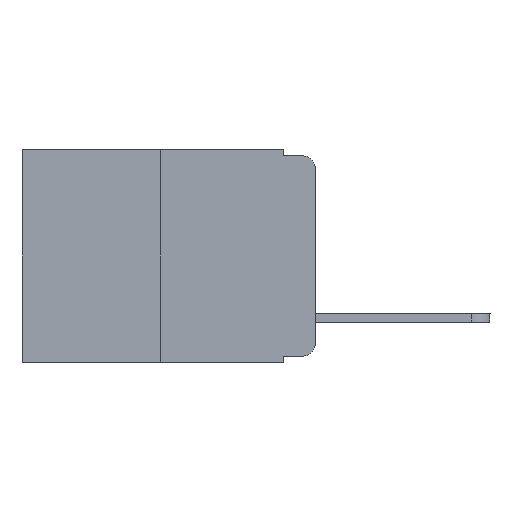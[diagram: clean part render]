
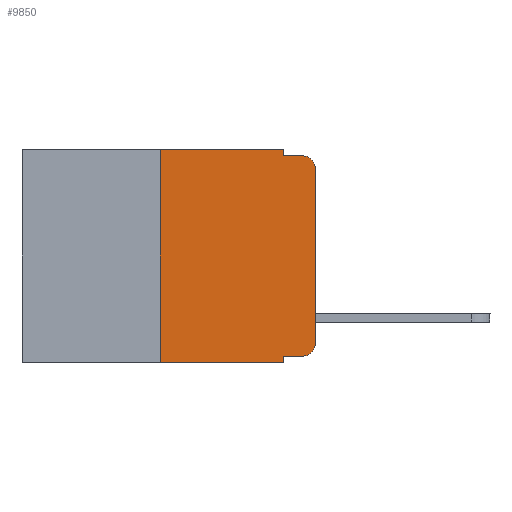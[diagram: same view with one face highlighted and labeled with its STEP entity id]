
A CAD part, left-side view. The second image highlights one B-rep face of the part: STEP entity #9850.
In plain terms, the highlighted planar face has unit normal (-1, 0, 0).
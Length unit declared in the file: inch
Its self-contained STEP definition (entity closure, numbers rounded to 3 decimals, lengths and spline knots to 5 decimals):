
#10 = ORIENTED_EDGE ( 'NONE', *, *, #16839, .T. ) ;
#225 = ORIENTED_EDGE ( 'NONE', *, *, #1136, .F. ) ;
#722 = CARTESIAN_POINT ( 'NONE',  ( 0., 0.02, -0.313 ) ) ;
#817 = DIRECTION ( 'NONE',  ( 0., 0., -1. ) ) ;
#880 = ORIENTED_EDGE ( 'NONE', *, *, #20250, .F. ) ;
#1073 = CARTESIAN_POINT ( 'NONE',  ( 0., 0., -0.313 ) ) ;
#1102 = EDGE_CURVE ( 'NONE', #17290, #2935, #16738, .T. ) ;
#1136 = EDGE_CURVE ( 'NONE', #17198, #19811, #17322, .T. ) ;
#1626 = VECTOR ( 'NONE', #12960, 39.37008 ) ;
#1809 = DIRECTION ( 'NONE',  ( 0., 0., -1. ) ) ;
#1826 = VERTEX_POINT ( 'NONE', #2982 ) ;
#2339 = CARTESIAN_POINT ( 'NONE',  ( 0., 0.051, -0.333 ) ) ;
#2357 = VECTOR ( 'NONE', #1809, 39.37008 ) ;
#2485 = EDGE_CURVE ( 'NONE', #13202, #9995, #9866, .T. ) ;
#2821 = EDGE_CURVE ( 'NONE', #19811, #8246, #12949, .T. ) ;
#2871 = AXIS2_PLACEMENT_3D ( 'NONE', #7156, #5715, #10146 ) ;
#2935 = VERTEX_POINT ( 'NONE', #4811 ) ;
#2982 = CARTESIAN_POINT ( 'NONE',  ( 0., 0.02, -0.333 ) ) ;
#3121 = CARTESIAN_POINT ( 'NONE',  ( 0., 0.051, -0.01 ) ) ;
#3383 = EDGE_CURVE ( 'NONE', #13202, #17198, #8589, .T. ) ;
#3696 = ORIENTED_EDGE ( 'NONE', *, *, #3383, .F. ) ;
#4072 = AXIS2_PLACEMENT_3D ( 'NONE', #7549, #15068, #19740 ) ;
#4455 = CIRCLE ( 'NONE', #16898, 0.02 ) ;
#4811 = CARTESIAN_POINT ( 'NONE',  ( 0., 0., -0.03 ) ) ;
#4824 = CARTESIAN_POINT ( 'NONE',  ( 0., 0.473, -0.343 ) ) ;
#4958 = LINE ( 'NONE', #11219, #12632 ) ;
#5237 = VECTOR ( 'NONE', #817, 39.37008 ) ;
#5255 = ORIENTED_EDGE ( 'NONE', *, *, #5958, .T. ) ;
#5276 = VECTOR ( 'NONE', #18372, 39.37008 ) ;
#5350 = LINE ( 'NONE', #2339, #8603 ) ;
#5715 = DIRECTION ( 'NONE',  ( -1., 0., 0. ) ) ;
#5958 = EDGE_CURVE ( 'NONE', #2935, #11087, #12752, .T. ) ;
#7139 = CARTESIAN_POINT ( 'NONE',  ( 0., 0.25, -0.343 ) ) ;
#7156 = CARTESIAN_POINT ( 'NONE',  ( 0., 0.02, -0.03 ) ) ;
#7549 = CARTESIAN_POINT ( 'NONE',  ( 0., 0.473, 0. ) ) ;
#8246 = VERTEX_POINT ( 'NONE', #3121 ) ;
#8589 = LINE ( 'NONE', #13322, #9729 ) ;
#8603 = VECTOR ( 'NONE', #14796, 39.37008 ) ;
#8794 = FACE_OUTER_BOUND ( 'NONE', #15104, .T. ) ;
#8991 = PLANE ( 'NONE',  #4072 ) ;
#9330 = CARTESIAN_POINT ( 'NONE',  ( 0., 0.473, 0. ) ) ;
#9729 = VECTOR ( 'NONE', #16395, 39.37008 ) ;
#9737 = CARTESIAN_POINT ( 'NONE',  ( 0., 0.051, 0. ) ) ;
#9850 = ADVANCED_FACE ( 'NONE', ( #8794 ), #8991, .F. ) ;
#9866 = LINE ( 'NONE', #4824, #1626 ) ;
#9995 = VERTEX_POINT ( 'NONE', #17470 ) ;
#10096 = DIRECTION ( 'NONE',  ( 0., 0., -1. ) ) ;
#10146 = DIRECTION ( 'NONE',  ( 0., 0., -1. ) ) ;
#10459 = EDGE_CURVE ( 'NONE', #14289, #1826, #5350, .T. ) ;
#10477 = CARTESIAN_POINT ( 'NONE',  ( 0., 0.02, -0.01 ) ) ;
#11087 = VERTEX_POINT ( 'NONE', #10477 ) ;
#11219 = CARTESIAN_POINT ( 'NONE',  ( 0., 0.051, -0.01 ) ) ;
#11792 = EDGE_CURVE ( 'NONE', #8246, #11087, #4958, .T. ) ;
#11809 = CARTESIAN_POINT ( 'NONE',  ( 0., 0.25, 0. ) ) ;
#12170 = VECTOR ( 'NONE', #18967, 39.37008 ) ;
#12632 = VECTOR ( 'NONE', #17448, 39.37008 ) ;
#12752 = CIRCLE ( 'NONE', #2871, 0.02 ) ;
#12949 = LINE ( 'NONE', #9737, #2357 ) ;
#12960 = DIRECTION ( 'NONE',  ( 0., -1., 0. ) ) ;
#12989 = CARTESIAN_POINT ( 'NONE',  ( 0., 0.051, 0. ) ) ;
#13202 = VERTEX_POINT ( 'NONE', #7139 ) ;
#13322 = CARTESIAN_POINT ( 'NONE',  ( 0., 0.25, 0. ) ) ;
#14289 = VERTEX_POINT ( 'NONE', #15868 ) ;
#14796 = DIRECTION ( 'NONE',  ( 0., -1., 0. ) ) ;
#15068 = DIRECTION ( 'NONE',  ( 1., 0., 0. ) ) ;
#15104 = EDGE_LOOP ( 'NONE', ( #16625, #5255, #18256, #19134, #225, #3696, #16570, #880, #18058, #10 ) ) ;
#15868 = CARTESIAN_POINT ( 'NONE',  ( 0., 0.051, -0.333 ) ) ;
#16395 = DIRECTION ( 'NONE',  ( 0., 0., 1. ) ) ;
#16548 = LINE ( 'NONE', #12989, #5237 ) ;
#16570 = ORIENTED_EDGE ( 'NONE', *, *, #2485, .T. ) ;
#16625 = ORIENTED_EDGE ( 'NONE', *, *, #1102, .T. ) ;
#16738 = LINE ( 'NONE', #19888, #5276 ) ;
#16839 = EDGE_CURVE ( 'NONE', #1826, #17290, #4455, .T. ) ;
#16898 = AXIS2_PLACEMENT_3D ( 'NONE', #722, #19309, #10096 ) ;
#17198 = VERTEX_POINT ( 'NONE', #11809 ) ;
#17290 = VERTEX_POINT ( 'NONE', #1073 ) ;
#17322 = LINE ( 'NONE', #9330, #12170 ) ;
#17448 = DIRECTION ( 'NONE',  ( 0., -1., 0. ) ) ;
#17470 = CARTESIAN_POINT ( 'NONE',  ( 0., 0.051, -0.343 ) ) ;
#18058 = ORIENTED_EDGE ( 'NONE', *, *, #10459, .T. ) ;
#18098 = CARTESIAN_POINT ( 'NONE',  ( 0., 0.051, 0. ) ) ;
#18256 = ORIENTED_EDGE ( 'NONE', *, *, #11792, .F. ) ;
#18372 = DIRECTION ( 'NONE',  ( 0., 0., 1. ) ) ;
#18967 = DIRECTION ( 'NONE',  ( 0., -1., 0. ) ) ;
#19134 = ORIENTED_EDGE ( 'NONE', *, *, #2821, .F. ) ;
#19309 = DIRECTION ( 'NONE',  ( -1., 0., 0. ) ) ;
#19740 = DIRECTION ( 'NONE',  ( 0., 0., -1. ) ) ;
#19811 = VERTEX_POINT ( 'NONE', #18098 ) ;
#19888 = CARTESIAN_POINT ( 'NONE',  ( 0., 0., 0. ) ) ;
#20250 = EDGE_CURVE ( 'NONE', #14289, #9995, #16548, .T. ) ;
